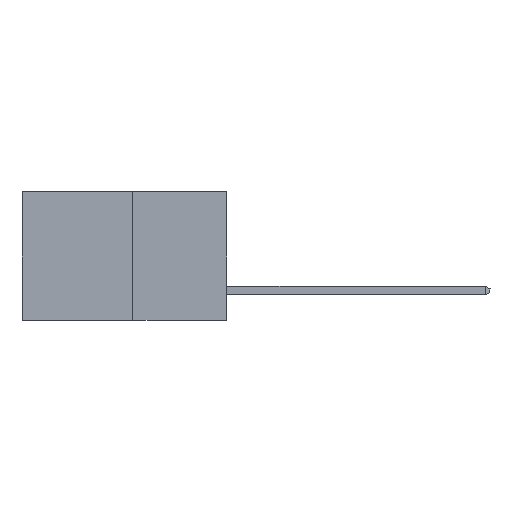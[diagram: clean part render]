
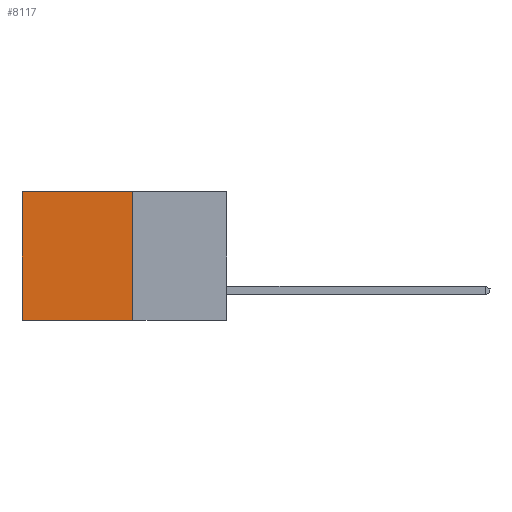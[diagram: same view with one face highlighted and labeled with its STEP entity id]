
A CAD part, left-side view. The second image highlights one B-rep face of the part: STEP entity #8117.
In plain terms, the highlighted planar face has unit normal (-1, 0, 0).
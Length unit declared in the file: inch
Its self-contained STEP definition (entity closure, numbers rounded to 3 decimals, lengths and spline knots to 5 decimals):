
#128 = PLANE ( 'NONE',  #4432 ) ;
#166 = CARTESIAN_POINT ( 'NONE',  ( 0.277, 0.27, -0.37 ) ) ;
#826 = DIRECTION ( 'NONE',  ( 0., 1., 0. ) ) ;
#931 = EDGE_CURVE ( 'NONE', #5502, #1255, #6309, .T. ) ;
#1077 = DIRECTION ( 'NONE',  ( 0., 0., -1. ) ) ;
#1168 = CARTESIAN_POINT ( 'NONE',  ( 0.277, 0.59, -0.37 ) ) ;
#1255 = VERTEX_POINT ( 'NONE', #1508 ) ;
#1361 = VERTEX_POINT ( 'NONE', #6537 ) ;
#1508 = CARTESIAN_POINT ( 'NONE',  ( 0.277, 0.59, 0. ) ) ;
#1559 = VECTOR ( 'NONE', #1077, 39.37008 ) ;
#1782 = FACE_OUTER_BOUND ( 'NONE', #5289, .T. ) ;
#2470 = DIRECTION ( 'NONE',  ( 1., 0., 0. ) ) ;
#2872 = DIRECTION ( 'NONE',  ( 0., 0., -1. ) ) ;
#3254 = LINE ( 'NONE', #7513, #9384 ) ;
#3863 = LINE ( 'NONE', #1168, #1559 ) ;
#4252 = VECTOR ( 'NONE', #826, 39.37008 ) ;
#4418 = CARTESIAN_POINT ( 'NONE',  ( 0.277, 0.27, 0. ) ) ;
#4432 = AXIS2_PLACEMENT_3D ( 'NONE', #4725, #2470, #7894 ) ;
#4725 = CARTESIAN_POINT ( 'NONE',  ( 0.277, 0.27, -0.37 ) ) ;
#4732 = VERTEX_POINT ( 'NONE', #166 ) ;
#5289 = EDGE_LOOP ( 'NONE', ( #6466, #9264, #6490, #7812 ) ) ;
#5502 = VERTEX_POINT ( 'NONE', #9514 ) ;
#5594 = EDGE_CURVE ( 'NONE', #4732, #1361, #6074, .T. ) ;
#6074 = LINE ( 'NONE', #9147, #9873 ) ;
#6309 = LINE ( 'NONE', #4418, #4252 ) ;
#6466 = ORIENTED_EDGE ( 'NONE', *, *, #7260, .T. ) ;
#6490 = ORIENTED_EDGE ( 'NONE', *, *, #8263, .F. ) ;
#6537 = CARTESIAN_POINT ( 'NONE',  ( 0.277, 0.59, -0.37 ) ) ;
#7260 = EDGE_CURVE ( 'NONE', #1255, #1361, #3863, .T. ) ;
#7513 = CARTESIAN_POINT ( 'NONE',  ( 0.277, 0.27, -0.37 ) ) ;
#7812 = ORIENTED_EDGE ( 'NONE', *, *, #931, .T. ) ;
#7894 = DIRECTION ( 'NONE',  ( 0., 0., -1. ) ) ;
#8117 = ADVANCED_FACE ( 'NONE', ( #1782 ), #128, .F. ) ;
#8263 = EDGE_CURVE ( 'NONE', #5502, #4732, #3254, .T. ) ;
#8933 = DIRECTION ( 'NONE',  ( 0., 1., 0. ) ) ;
#9147 = CARTESIAN_POINT ( 'NONE',  ( 0.277, 0.27, -0.37 ) ) ;
#9264 = ORIENTED_EDGE ( 'NONE', *, *, #5594, .F. ) ;
#9384 = VECTOR ( 'NONE', #2872, 39.37008 ) ;
#9514 = CARTESIAN_POINT ( 'NONE',  ( 0.277, 0.27, 0. ) ) ;
#9873 = VECTOR ( 'NONE', #8933, 39.37008 ) ;
